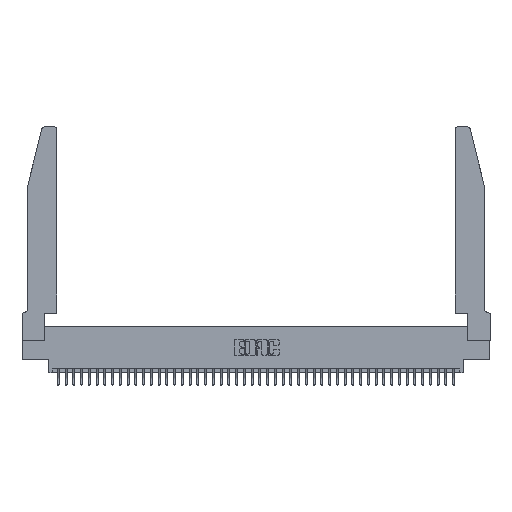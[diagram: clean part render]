
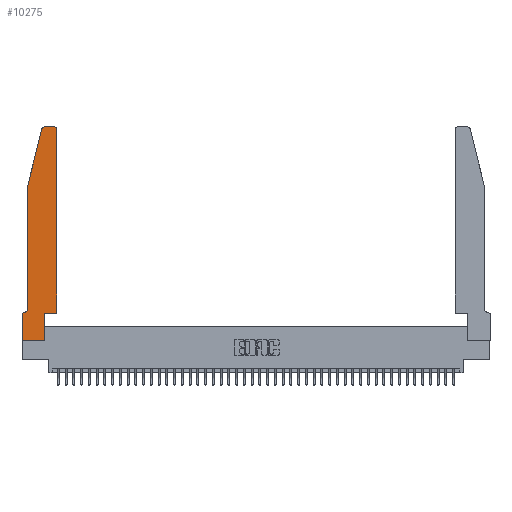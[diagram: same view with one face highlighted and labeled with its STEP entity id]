
A CAD part, top view. The second image highlights one B-rep face of the part: STEP entity #10275.
In plain terms, the highlighted planar face has unit normal (0, 0, 1).
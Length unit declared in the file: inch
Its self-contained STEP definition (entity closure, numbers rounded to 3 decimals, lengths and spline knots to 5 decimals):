
#248 = ORIENTED_EDGE ( 'NONE', *, *, #17135, .T. ) ;
#270 = CARTESIAN_POINT ( 'NONE',  ( 0.0755, 0.35, 0.37 ) ) ;
#459 = VERTEX_POINT ( 'NONE', #21119 ) ;
#846 = LINE ( 'NONE', #5992, #36451 ) ;
#1144 = EDGE_CURVE ( 'NONE', #1384, #21233, #31154, .T. ) ;
#1156 = ORIENTED_EDGE ( 'NONE', *, *, #1144, .T. ) ;
#1384 = VERTEX_POINT ( 'NONE', #10686 ) ;
#1566 = DIRECTION ( 'NONE',  ( 0., 0., 1. ) ) ;
#1573 = VERTEX_POINT ( 'NONE', #22027 ) ;
#2262 = LINE ( 'NONE', #6653, #28776 ) ;
#2537 = VERTEX_POINT ( 'NONE', #34417 ) ;
#2655 = CARTESIAN_POINT ( 'NONE',  ( 0.4205, 2.72, 0.37 ) ) ;
#2682 = AXIS2_PLACEMENT_3D ( 'NONE', #4962, #29159, #8412 ) ;
#3058 = ORIENTED_EDGE ( 'NONE', *, *, #3657, .T. ) ;
#3322 = DIRECTION ( 'NONE',  ( 1., 0., 0. ) ) ;
#3657 = EDGE_CURVE ( 'NONE', #27904, #22732, #14215, .T. ) ;
#3928 = EDGE_CURVE ( 'NONE', #459, #1573, #2262, .T. ) ;
#4962 = CARTESIAN_POINT ( 'NONE',  ( 0.284, 2.72, 0.37 ) ) ;
#5926 = EDGE_CURVE ( 'NONE', #21233, #26089, #43878, .T. ) ;
#5992 = CARTESIAN_POINT ( 'NONE',  ( 0., 0., 0.37 ) ) ;
#6119 = DIRECTION ( 'NONE',  ( 1., 0., 0. ) ) ;
#6653 = CARTESIAN_POINT ( 'NONE',  ( 0.0755, 2., 0.37 ) ) ;
#7411 = EDGE_CURVE ( 'NONE', #31901, #39807, #32523, .T. ) ;
#8412 = DIRECTION ( 'NONE',  ( 1., 0., 0. ) ) ;
#9112 = VECTOR ( 'NONE', #30074, 39.37008 ) ;
#10275 = ADVANCED_FACE ( 'NONE', ( #22698 ), #39422, .T. ) ;
#10290 = VECTOR ( 'NONE', #24480, 39.37008 ) ;
#10686 = CARTESIAN_POINT ( 'NONE',  ( 0.4505, 2.72, 0.37 ) ) ;
#10921 = LINE ( 'NONE', #27130, #20123 ) ;
#11630 = ORIENTED_EDGE ( 'NONE', *, *, #40138, .T. ) ;
#11653 = EDGE_CURVE ( 'NONE', #2537, #1384, #10921, .T. ) ;
#12004 = CARTESIAN_POINT ( 'NONE',  ( 0.0055, 0.42, 0.37 ) ) ;
#13364 = EDGE_CURVE ( 'NONE', #1573, #27904, #18368, .T. ) ;
#14172 = VECTOR ( 'NONE', #3322, 39.37008 ) ;
#14215 = CIRCLE ( 'NONE', #31396, 0.07 ) ;
#14314 = CARTESIAN_POINT ( 'NONE',  ( 0., 0.35, 0.37 ) ) ;
#14371 = ORIENTED_EDGE ( 'NONE', *, *, #7411, .T. ) ;
#15521 = DIRECTION ( 'NONE',  ( -1., 0., 0. ) ) ;
#16462 = VECTOR ( 'NONE', #44170, 39.37008 ) ;
#17135 = EDGE_CURVE ( 'NONE', #27049, #2537, #36886, .T. ) ;
#17201 = ORIENTED_EDGE ( 'NONE', *, *, #5926, .T. ) ;
#18229 = VERTEX_POINT ( 'NONE', #14314 ) ;
#18361 = ORIENTED_EDGE ( 'NONE', *, *, #3928, .T. ) ;
#18368 = LINE ( 'NONE', #40387, #9112 ) ;
#20123 = VECTOR ( 'NONE', #20372, 39.37008 ) ;
#20372 = DIRECTION ( 'NONE',  ( 0., 1., 0. ) ) ;
#20900 = CARTESIAN_POINT ( 'NONE',  ( 0.2865, 0., 0.37 ) ) ;
#21119 = CARTESIAN_POINT ( 'NONE',  ( 0.25487, 2.72718, 0.37 ) ) ;
#21233 = VERTEX_POINT ( 'NONE', #33677 ) ;
#21864 = ORIENTED_EDGE ( 'NONE', *, *, #11653, .T. ) ;
#22027 = CARTESIAN_POINT ( 'NONE',  ( 0.0755, 2., 0.37 ) ) ;
#22197 = CARTESIAN_POINT ( 'NONE',  ( 0., 0., 0.37 ) ) ;
#22698 = FACE_OUTER_BOUND ( 'NONE', #26238, .T. ) ;
#22732 = VERTEX_POINT ( 'NONE', #36679 ) ;
#24480 = DIRECTION ( 'NONE',  ( -1., 0., 0. ) ) ;
#24685 = LINE ( 'NONE', #28442, #41815 ) ;
#25793 = DIRECTION ( 'NONE',  ( 1., 0., 0. ) ) ;
#26089 = VERTEX_POINT ( 'NONE', #31784 ) ;
#26238 = EDGE_LOOP ( 'NONE', ( #17201, #37681, #18361, #32200, #3058, #44504, #26915, #14371, #11630, #248, #21864, #1156 ) ) ;
#26688 = VECTOR ( 'NONE', #32949, 39.37008 ) ;
#26845 = DIRECTION ( 'NONE',  ( 0., 0., 1. ) ) ;
#26915 = ORIENTED_EDGE ( 'NONE', *, *, #36338, .T. ) ;
#27049 = VERTEX_POINT ( 'NONE', #36326 ) ;
#27130 = CARTESIAN_POINT ( 'NONE',  ( 0.4505, 0.35, 0.37 ) ) ;
#27419 = CARTESIAN_POINT ( 'NONE',  ( 0.0755, 0.42, 0.37 ) ) ;
#27904 = VERTEX_POINT ( 'NONE', #27419 ) ;
#28442 = CARTESIAN_POINT ( 'NONE',  ( 0.2865, 0.35, 0.37 ) ) ;
#28776 = VECTOR ( 'NONE', #34300, 39.37008 ) ;
#28931 = EDGE_CURVE ( 'NONE', #26089, #459, #41191, .T. ) ;
#29159 = DIRECTION ( 'NONE',  ( 0., 0., 1. ) ) ;
#30074 = DIRECTION ( 'NONE',  ( 0., -1., 0. ) ) ;
#30202 = DIRECTION ( 'NONE',  ( 0., -1., 0. ) ) ;
#31014 = AXIS2_PLACEMENT_3D ( 'NONE', #32513, #1566, #25793 ) ;
#31154 = CIRCLE ( 'NONE', #44209, 0.03 ) ;
#31396 = AXIS2_PLACEMENT_3D ( 'NONE', #12004, #36132, #15521 ) ;
#31784 = CARTESIAN_POINT ( 'NONE',  ( 0.284, 2.75, 0.37 ) ) ;
#31901 = VERTEX_POINT ( 'NONE', #22197 ) ;
#32200 = ORIENTED_EDGE ( 'NONE', *, *, #13364, .T. ) ;
#32513 = CARTESIAN_POINT ( 'NONE',  ( 0., 0.35, 0.37 ) ) ;
#32523 = LINE ( 'NONE', #44583, #14172 ) ;
#32800 = CARTESIAN_POINT ( 'NONE',  ( 0.4505, 0.35, 0.37 ) ) ;
#32949 = DIRECTION ( 'NONE',  ( 1., 0., 0. ) ) ;
#33579 = EDGE_CURVE ( 'NONE', #22732, #18229, #36702, .T. ) ;
#33677 = CARTESIAN_POINT ( 'NONE',  ( 0.4205, 2.75, 0.37 ) ) ;
#34300 = DIRECTION ( 'NONE',  ( -0.239, -0.971, 0. ) ) ;
#34417 = CARTESIAN_POINT ( 'NONE',  ( 0.4505, 0.35, 0.37 ) ) ;
#36132 = DIRECTION ( 'NONE',  ( 0., 0., -1. ) ) ;
#36326 = CARTESIAN_POINT ( 'NONE',  ( 0.2865, 0.35, 0.37 ) ) ;
#36338 = EDGE_CURVE ( 'NONE', #18229, #31901, #846, .T. ) ;
#36451 = VECTOR ( 'NONE', #30202, 39.37008 ) ;
#36679 = CARTESIAN_POINT ( 'NONE',  ( 0.0055, 0.35, 0.37 ) ) ;
#36702 = LINE ( 'NONE', #270, #10290 ) ;
#36886 = LINE ( 'NONE', #32800, #26688 ) ;
#37681 = ORIENTED_EDGE ( 'NONE', *, *, #28931, .T. ) ;
#39422 = PLANE ( 'NONE',  #31014 ) ;
#39807 = VERTEX_POINT ( 'NONE', #20900 ) ;
#40138 = EDGE_CURVE ( 'NONE', #39807, #27049, #24685, .T. ) ;
#40387 = CARTESIAN_POINT ( 'NONE',  ( 0.0755, 2., 0.37 ) ) ;
#40734 = CARTESIAN_POINT ( 'NONE',  ( 0.2605, 2.75, 0.37 ) ) ;
#41191 = CIRCLE ( 'NONE', #2682, 0.03 ) ;
#41815 = VECTOR ( 'NONE', #42215, 39.37008 ) ;
#42215 = DIRECTION ( 'NONE',  ( 0., 1., 0. ) ) ;
#43878 = LINE ( 'NONE', #40734, #16462 ) ;
#44170 = DIRECTION ( 'NONE',  ( -1., 0., 0. ) ) ;
#44209 = AXIS2_PLACEMENT_3D ( 'NONE', #2655, #26845, #6119 ) ;
#44504 = ORIENTED_EDGE ( 'NONE', *, *, #33579, .T. ) ;
#44583 = CARTESIAN_POINT ( 'NONE',  ( 0., 0., 0.37 ) ) ;
